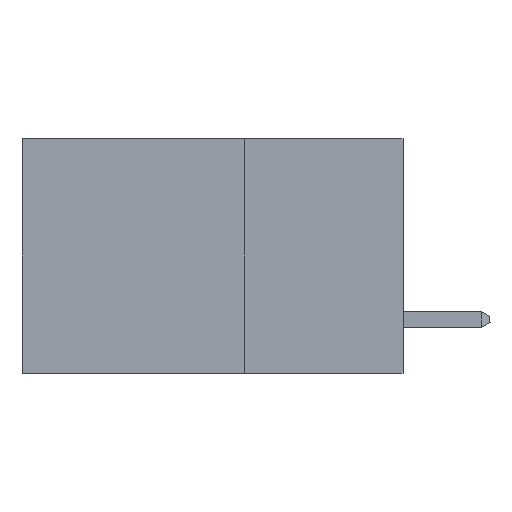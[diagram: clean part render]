
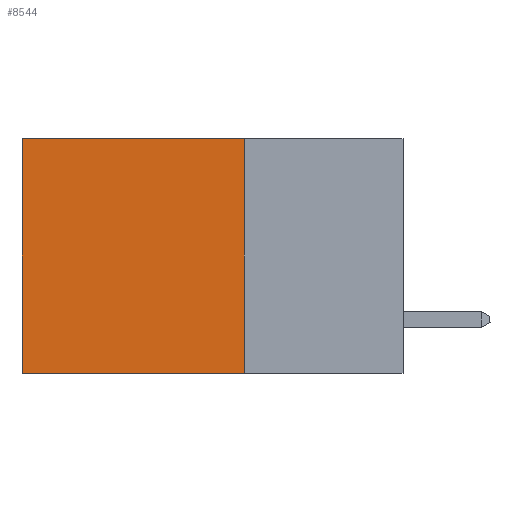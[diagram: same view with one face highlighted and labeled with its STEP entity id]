
A CAD part, left-side view. The second image highlights one B-rep face of the part: STEP entity #8544.
In plain terms, the highlighted planar face has unit normal (-1, 0, 0).
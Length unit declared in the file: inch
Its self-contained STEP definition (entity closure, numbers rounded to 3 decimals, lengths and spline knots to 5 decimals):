
#1440 = EDGE_LOOP ( 'NONE', ( #7683, #2693, #12232, #12523 ) ) ;
#1769 = DIRECTION ( 'NONE',  ( 1., 0., 0. ) ) ;
#2412 = DIRECTION ( 'NONE',  ( 0., 0., -1. ) ) ;
#2615 = CARTESIAN_POINT ( 'NONE',  ( 0.2875, 0.25, -0.37 ) ) ;
#2687 = FACE_OUTER_BOUND ( 'NONE', #1440, .T. ) ;
#2693 = ORIENTED_EDGE ( 'NONE', *, *, #4194, .F. ) ;
#3246 = VERTEX_POINT ( 'NONE', #12568 ) ;
#3339 = VERTEX_POINT ( 'NONE', #9655 ) ;
#3725 = EDGE_CURVE ( 'NONE', #3246, #13276, #13685, .T. ) ;
#4066 = DIRECTION ( 'NONE',  ( 0., 0., -1. ) ) ;
#4194 = EDGE_CURVE ( 'NONE', #13276, #5472, #8171, .T. ) ;
#4692 = VECTOR ( 'NONE', #9930, 39.37008 ) ;
#5006 = CARTESIAN_POINT ( 'NONE',  ( 0.2875, 0.25, -0.37 ) ) ;
#5472 = VERTEX_POINT ( 'NONE', #9852 ) ;
#5938 = EDGE_CURVE ( 'NONE', #3339, #5472, #9255, .T. ) ;
#7141 = DIRECTION ( 'NONE',  ( 0., 0., -1. ) ) ;
#7634 = EDGE_CURVE ( 'NONE', #3246, #3339, #11352, .T. ) ;
#7683 = ORIENTED_EDGE ( 'NONE', *, *, #5938, .T. ) ;
#8171 = LINE ( 'NONE', #2615, #4692 ) ;
#8241 = CARTESIAN_POINT ( 'NONE',  ( 0.2875, 0.25, 0. ) ) ;
#8520 = VECTOR ( 'NONE', #9097, 39.37008 ) ;
#8544 = ADVANCED_FACE ( 'NONE', ( #2687 ), #13495, .F. ) ;
#9097 = DIRECTION ( 'NONE',  ( 0., 1., 0. ) ) ;
#9245 = AXIS2_PLACEMENT_3D ( 'NONE', #8241, #1769, #7141 ) ;
#9255 = LINE ( 'NONE', #10852, #11589 ) ;
#9387 = CARTESIAN_POINT ( 'NONE',  ( 0.2875, 0.25, 0. ) ) ;
#9655 = CARTESIAN_POINT ( 'NONE',  ( 0.2875, 0.6, 0. ) ) ;
#9852 = CARTESIAN_POINT ( 'NONE',  ( 0.2875, 0.6, -0.37 ) ) ;
#9885 = VECTOR ( 'NONE', #4066, 39.37008 ) ;
#9930 = DIRECTION ( 'NONE',  ( 0., 1., 0. ) ) ;
#10852 = CARTESIAN_POINT ( 'NONE',  ( 0.2875, 0.6, 0. ) ) ;
#11352 = LINE ( 'NONE', #12484, #8520 ) ;
#11589 = VECTOR ( 'NONE', #2412, 39.37008 ) ;
#12232 = ORIENTED_EDGE ( 'NONE', *, *, #3725, .F. ) ;
#12484 = CARTESIAN_POINT ( 'NONE',  ( 0.2875, 0.25, 0. ) ) ;
#12523 = ORIENTED_EDGE ( 'NONE', *, *, #7634, .T. ) ;
#12568 = CARTESIAN_POINT ( 'NONE',  ( 0.2875, 0.25, 0. ) ) ;
#13276 = VERTEX_POINT ( 'NONE', #5006 ) ;
#13495 = PLANE ( 'NONE',  #9245 ) ;
#13685 = LINE ( 'NONE', #9387, #9885 ) ;
